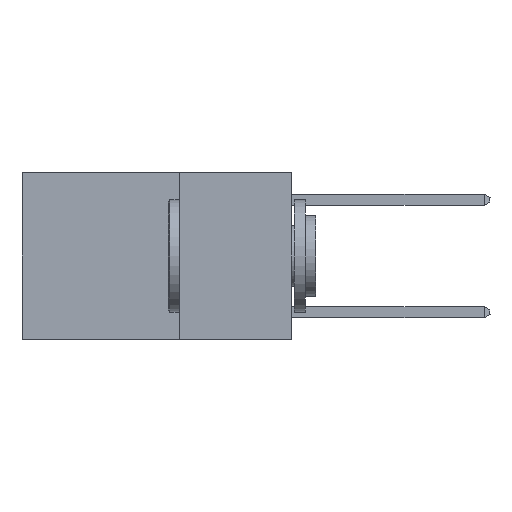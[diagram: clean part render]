
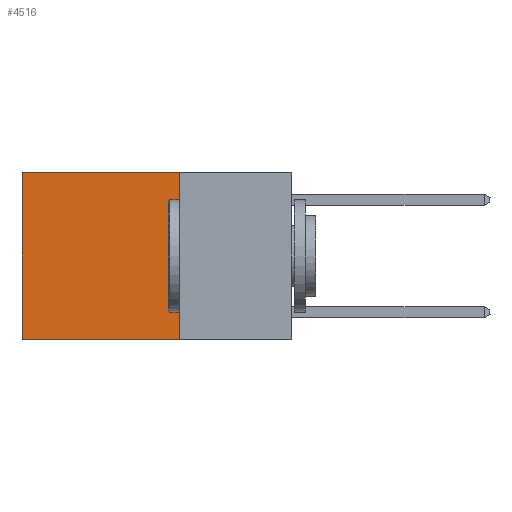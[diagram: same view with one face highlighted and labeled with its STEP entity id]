
A CAD part, left-side view. The second image highlights one B-rep face of the part: STEP entity #4516.
In plain terms, the highlighted planar face has unit normal (-1, 0, 0).
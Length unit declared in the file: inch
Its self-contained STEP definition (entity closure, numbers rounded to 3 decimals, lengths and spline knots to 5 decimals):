
#305 = VERTEX_POINT ( 'NONE', #13871 ) ;
#572 = CARTESIAN_POINT ( 'NONE',  ( 0.2625, 0.6, 0. ) ) ;
#790 = ORIENTED_EDGE ( 'NONE', *, *, #4664, .F. ) ;
#832 = CARTESIAN_POINT ( 'NONE',  ( 0.2625, 0.25, 0. ) ) ;
#2267 = CARTESIAN_POINT ( 'NONE',  ( 0.2625, 0.25, 0. ) ) ;
#2606 = ORIENTED_EDGE ( 'NONE', *, *, #3524, .T. ) ;
#2834 = VECTOR ( 'NONE', #4686, 39.37008 ) ;
#3524 = EDGE_CURVE ( 'NONE', #8915, #5341, #13528, .T. ) ;
#4516 = ADVANCED_FACE ( 'NONE', ( #9448 ), #11100, .F. ) ;
#4664 = EDGE_CURVE ( 'NONE', #305, #5341, #8837, .T. ) ;
#4686 = DIRECTION ( 'NONE',  ( 0., 1., 0. ) ) ;
#5216 = VECTOR ( 'NONE', #11035, 39.37008 ) ;
#5341 = VERTEX_POINT ( 'NONE', #15664 ) ;
#6225 = CARTESIAN_POINT ( 'NONE',  ( 0.2625, 0.25, 0. ) ) ;
#6761 = CARTESIAN_POINT ( 'NONE',  ( 0.2625, 0.6, 0. ) ) ;
#6851 = DIRECTION ( 'NONE',  ( 0., 0., -1. ) ) ;
#7500 = LINE ( 'NONE', #6225, #12815 ) ;
#7545 = DIRECTION ( 'NONE',  ( 1., 0., 0. ) ) ;
#8837 = LINE ( 'NONE', #12464, #2834 ) ;
#8915 = VERTEX_POINT ( 'NONE', #572 ) ;
#9448 = FACE_OUTER_BOUND ( 'NONE', #9554, .T. ) ;
#9554 = EDGE_LOOP ( 'NONE', ( #2606, #790, #11669, #11357 ) ) ;
#10618 = AXIS2_PLACEMENT_3D ( 'NONE', #11197, #7545, #16292 ) ;
#11035 = DIRECTION ( 'NONE',  ( 0., 1., 0. ) ) ;
#11100 = PLANE ( 'NONE',  #10618 ) ;
#11197 = CARTESIAN_POINT ( 'NONE',  ( 0.2625, 0.25, 0. ) ) ;
#11357 = ORIENTED_EDGE ( 'NONE', *, *, #15544, .T. ) ;
#11410 = VECTOR ( 'NONE', #6851, 39.37008 ) ;
#11576 = DIRECTION ( 'NONE',  ( 0., 0., -1. ) ) ;
#11669 = ORIENTED_EDGE ( 'NONE', *, *, #15186, .F. ) ;
#12464 = CARTESIAN_POINT ( 'NONE',  ( 0.2625, 0.25, -0.37 ) ) ;
#12815 = VECTOR ( 'NONE', #11576, 39.37008 ) ;
#13528 = LINE ( 'NONE', #6761, #11410 ) ;
#13818 = LINE ( 'NONE', #2267, #5216 ) ;
#13871 = CARTESIAN_POINT ( 'NONE',  ( 0.2625, 0.25, -0.37 ) ) ;
#15012 = VERTEX_POINT ( 'NONE', #832 ) ;
#15186 = EDGE_CURVE ( 'NONE', #15012, #305, #7500, .T. ) ;
#15544 = EDGE_CURVE ( 'NONE', #15012, #8915, #13818, .T. ) ;
#15664 = CARTESIAN_POINT ( 'NONE',  ( 0.2625, 0.6, -0.37 ) ) ;
#16292 = DIRECTION ( 'NONE',  ( 0., 0., -1. ) ) ;
